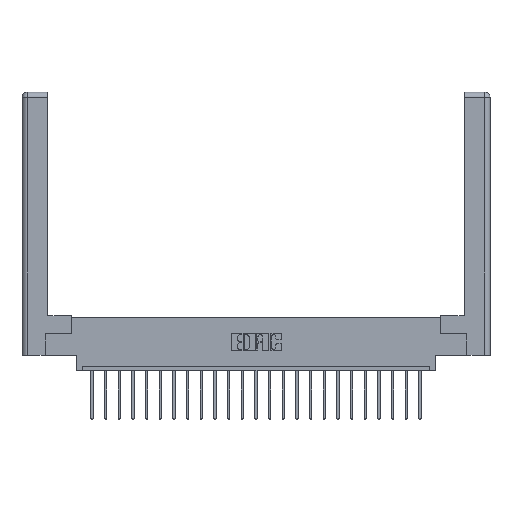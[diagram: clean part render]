
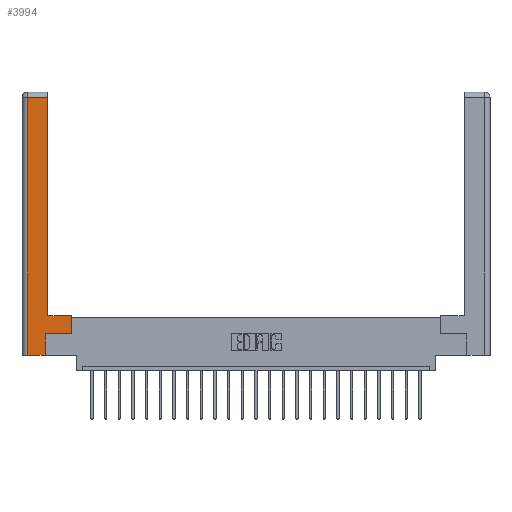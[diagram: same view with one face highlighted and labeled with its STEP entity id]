
A CAD part, top view. The second image highlights one B-rep face of the part: STEP entity #3994.
In plain terms, the highlighted planar face has unit normal (0, 0, 1).
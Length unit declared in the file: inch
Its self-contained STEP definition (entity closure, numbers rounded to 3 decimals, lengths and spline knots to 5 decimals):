
#217 = EDGE_CURVE ( 'NONE', #7626, #17435, #4668, .T. ) ;
#751 = CARTESIAN_POINT ( 'NONE',  ( 0.265, 0., 0. ) ) ;
#813 = DIRECTION ( 'NONE',  ( 1., 0., 0. ) ) ;
#946 = CARTESIAN_POINT ( 'NONE',  ( 0.295, 2.94, 0. ) ) ;
#1512 = ORIENTED_EDGE ( 'NONE', *, *, #16893, .T. ) ;
#1940 = CARTESIAN_POINT ( 'NONE',  ( 0.565, 0.45, 0. ) ) ;
#2251 = EDGE_CURVE ( 'NONE', #6626, #8767, #6072, .T. ) ;
#2286 = DIRECTION ( 'NONE',  ( 0., -1., 0. ) ) ;
#2422 = DIRECTION ( 'NONE',  ( 1., 0., 0. ) ) ;
#3344 = DIRECTION ( 'NONE',  ( 0., 1., 0. ) ) ;
#3443 = CARTESIAN_POINT ( 'NONE',  ( 0.0615, 0., 0. ) ) ;
#3593 = AXIS2_PLACEMENT_3D ( 'NONE', #23136, #12287, #5047 ) ;
#3994 = ADVANCED_FACE ( 'NONE', ( #10608 ), #23057, .F. ) ;
#4021 = DIRECTION ( 'NONE',  ( 0., 1., 0. ) ) ;
#4467 = VECTOR ( 'NONE', #2286, 39.37008 ) ;
#4569 = CARTESIAN_POINT ( 'NONE',  ( 0.565, 0.45, 0. ) ) ;
#4668 = LINE ( 'NONE', #13821, #8914 ) ;
#5047 = DIRECTION ( 'NONE',  ( -1., 0., 0. ) ) ;
#5813 = CARTESIAN_POINT ( 'NONE',  ( 0.565, 0.245, 0. ) ) ;
#6072 = LINE ( 'NONE', #1940, #20361 ) ;
#6404 = ORIENTED_EDGE ( 'NONE', *, *, #11725, .T. ) ;
#6626 = VERTEX_POINT ( 'NONE', #5813 ) ;
#6773 = CARTESIAN_POINT ( 'NONE',  ( 0.295, 0.45, 0. ) ) ;
#6862 = ORIENTED_EDGE ( 'NONE', *, *, #217, .T. ) ;
#7626 = VERTEX_POINT ( 'NONE', #6773 ) ;
#8261 = VECTOR ( 'NONE', #3344, 39.37008 ) ;
#8273 = LINE ( 'NONE', #751, #21650 ) ;
#8320 = CARTESIAN_POINT ( 'NONE',  ( 0.265, 0., 0. ) ) ;
#8600 = ORIENTED_EDGE ( 'NONE', *, *, #22431, .T. ) ;
#8767 = VERTEX_POINT ( 'NONE', #4569 ) ;
#8914 = VECTOR ( 'NONE', #10362, 39.37008 ) ;
#9217 = EDGE_CURVE ( 'NONE', #21399, #18308, #23530, .T. ) ;
#9298 = CARTESIAN_POINT ( 'NONE',  ( 0.0615, 2.94, 0. ) ) ;
#9507 = EDGE_LOOP ( 'NONE', ( #6862, #22421, #11062, #15063, #6404, #1512, #14747, #8600 ) ) ;
#10362 = DIRECTION ( 'NONE',  ( 0., 1., 0. ) ) ;
#10500 = VERTEX_POINT ( 'NONE', #12259 ) ;
#10608 = FACE_OUTER_BOUND ( 'NONE', #9507, .T. ) ;
#10864 = EDGE_CURVE ( 'NONE', #17435, #21399, #15717, .T. ) ;
#11052 = LINE ( 'NONE', #13454, #17836 ) ;
#11062 = ORIENTED_EDGE ( 'NONE', *, *, #9217, .T. ) ;
#11612 = LINE ( 'NONE', #22826, #15851 ) ;
#11725 = EDGE_CURVE ( 'NONE', #14394, #10500, #13113, .T. ) ;
#12259 = CARTESIAN_POINT ( 'NONE',  ( 0.265, 0.245, 0. ) ) ;
#12287 = DIRECTION ( 'NONE',  ( 0., 0., -1. ) ) ;
#12493 = CARTESIAN_POINT ( 'NONE',  ( 0.265, 0.245, 0. ) ) ;
#12905 = VECTOR ( 'NONE', #20334, 39.37008 ) ;
#13113 = LINE ( 'NONE', #12493, #8261 ) ;
#13454 = CARTESIAN_POINT ( 'NONE',  ( 0.565, 0.245, 0. ) ) ;
#13821 = CARTESIAN_POINT ( 'NONE',  ( 0.295, 3., 0. ) ) ;
#13999 = DIRECTION ( 'NONE',  ( -1., 0., 0. ) ) ;
#14394 = VERTEX_POINT ( 'NONE', #8320 ) ;
#14747 = ORIENTED_EDGE ( 'NONE', *, *, #2251, .T. ) ;
#15063 = ORIENTED_EDGE ( 'NONE', *, *, #18527, .T. ) ;
#15717 = LINE ( 'NONE', #9298, #12905 ) ;
#15851 = VECTOR ( 'NONE', #13999, 39.37008 ) ;
#16893 = EDGE_CURVE ( 'NONE', #10500, #6626, #11052, .T. ) ;
#17435 = VERTEX_POINT ( 'NONE', #946 ) ;
#17836 = VECTOR ( 'NONE', #813, 39.37008 ) ;
#18308 = VERTEX_POINT ( 'NONE', #3443 ) ;
#18527 = EDGE_CURVE ( 'NONE', #18308, #14394, #8273, .T. ) ;
#20265 = CARTESIAN_POINT ( 'NONE',  ( 0.0615, 0., 0. ) ) ;
#20334 = DIRECTION ( 'NONE',  ( -1., 0., 0. ) ) ;
#20361 = VECTOR ( 'NONE', #4021, 39.37008 ) ;
#21246 = CARTESIAN_POINT ( 'NONE',  ( 0.0615, 2.94, 0. ) ) ;
#21399 = VERTEX_POINT ( 'NONE', #21246 ) ;
#21650 = VECTOR ( 'NONE', #2422, 39.37008 ) ;
#22421 = ORIENTED_EDGE ( 'NONE', *, *, #10864, .T. ) ;
#22431 = EDGE_CURVE ( 'NONE', #8767, #7626, #11612, .T. ) ;
#22826 = CARTESIAN_POINT ( 'NONE',  ( 0.295, 0.45, 0. ) ) ;
#23057 = PLANE ( 'NONE',  #3593 ) ;
#23136 = CARTESIAN_POINT ( 'NONE',  ( 0., 0., 0. ) ) ;
#23530 = LINE ( 'NONE', #20265, #4467 ) ;
